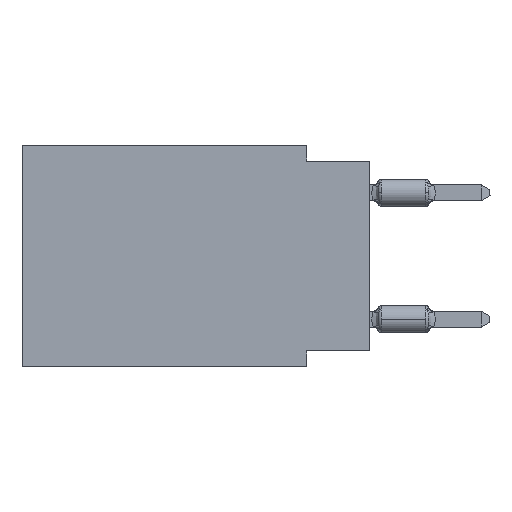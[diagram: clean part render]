
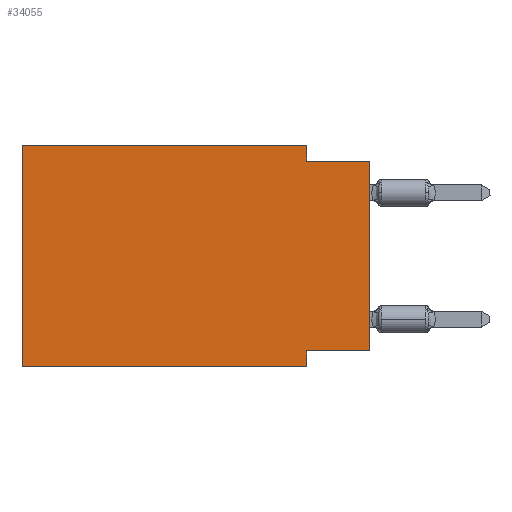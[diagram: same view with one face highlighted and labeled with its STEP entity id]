
A CAD part, left-side view. The second image highlights one B-rep face of the part: STEP entity #34055.
In plain terms, the highlighted planar face has unit normal (-1, 0, 0).
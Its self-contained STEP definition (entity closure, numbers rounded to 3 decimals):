
#623 = FACE_OUTER_BOUND ( 'NONE', #3907, .T. ) ;
#1321 = DIRECTION ( 'NONE',  ( 0., 0., -1. ) ) ;
#1369 = ORIENTED_EDGE ( 'NONE', *, *, #36295, .F. ) ;
#1447 = ORIENTED_EDGE ( 'NONE', *, *, #17365, .F. ) ;
#1953 = VERTEX_POINT ( 'NONE', #7689 ) ;
#2126 = DIRECTION ( 'NONE',  ( 0., 1., 0. ) ) ;
#2865 = VECTOR ( 'NONE', #28573, 1000. ) ;
#3158 = VERTEX_POINT ( 'NONE', #5037 ) ;
#3907 = EDGE_LOOP ( 'NONE', ( #31563, #3913, #12588, #1369, #12173, #6839, #1447, #6886 ) ) ;
#3913 = ORIENTED_EDGE ( 'NONE', *, *, #12245, .F. ) ;
#4157 = CARTESIAN_POINT ( 'NONE',  ( 0., 2.54, -0.635 ) ) ;
#4336 = LINE ( 'NONE', #18731, #15371 ) ;
#5037 = CARTESIAN_POINT ( 'NONE',  ( 0., 2.54, -8.255 ) ) ;
#5734 = LINE ( 'NONE', #35028, #26930 ) ;
#5789 = DIRECTION ( 'NONE',  ( 0., -1., 0. ) ) ;
#6024 = CARTESIAN_POINT ( 'NONE',  ( 0., 13.97, -8.89 ) ) ;
#6485 = CARTESIAN_POINT ( 'NONE',  ( 0., 0., 0. ) ) ;
#6839 = ORIENTED_EDGE ( 'NONE', *, *, #9500, .T. ) ;
#6886 = ORIENTED_EDGE ( 'NONE', *, *, #21259, .F. ) ;
#7689 = CARTESIAN_POINT ( 'NONE',  ( 0., 0., -0.635 ) ) ;
#7815 = EDGE_CURVE ( 'NONE', #43434, #20522, #46175, .T. ) ;
#9500 = EDGE_CURVE ( 'NONE', #43434, #27887, #12260, .T. ) ;
#9867 = DIRECTION ( 'NONE',  ( 0., 0., -1. ) ) ;
#10337 = LINE ( 'NONE', #28597, #28189 ) ;
#11064 = CARTESIAN_POINT ( 'NONE',  ( 0., 2.54, 0. ) ) ;
#12173 = ORIENTED_EDGE ( 'NONE', *, *, #7815, .F. ) ;
#12245 = EDGE_CURVE ( 'NONE', #22387, #1953, #4336, .T. ) ;
#12260 = LINE ( 'NONE', #6024, #30629 ) ;
#12588 = ORIENTED_EDGE ( 'NONE', *, *, #23973, .F. ) ;
#12964 = CARTESIAN_POINT ( 'NONE',  ( 0., 13.97, 0. ) ) ;
#15137 = LINE ( 'NONE', #11064, #46253 ) ;
#15371 = VECTOR ( 'NONE', #37236, 1000. ) ;
#17365 = EDGE_CURVE ( 'NONE', #3158, #27887, #10337, .T. ) ;
#18731 = CARTESIAN_POINT ( 'NONE',  ( 0., 0., -0.635 ) ) ;
#18931 = CARTESIAN_POINT ( 'NONE',  ( 0., 13.97, 0. ) ) ;
#20522 = VERTEX_POINT ( 'NONE', #18931 ) ;
#20640 = DIRECTION ( 'NONE',  ( 0., -1., 0. ) ) ;
#21259 = EDGE_CURVE ( 'NONE', #36828, #3158, #5734, .T. ) ;
#22072 = CARTESIAN_POINT ( 'NONE',  ( 0., 13.97, -8.89 ) ) ;
#22387 = VERTEX_POINT ( 'NONE', #4157 ) ;
#23973 = EDGE_CURVE ( 'NONE', #30638, #22387, #15137, .T. ) ;
#26930 = VECTOR ( 'NONE', #2126, 1000. ) ;
#27887 = VERTEX_POINT ( 'NONE', #29630 ) ;
#28189 = VECTOR ( 'NONE', #9867, 1000. ) ;
#28573 = DIRECTION ( 'NONE',  ( 0., 0., 1. ) ) ;
#28597 = CARTESIAN_POINT ( 'NONE',  ( 0., 2.54, -8.89 ) ) ;
#29630 = CARTESIAN_POINT ( 'NONE',  ( 0., 2.54, -8.89 ) ) ;
#30629 = VECTOR ( 'NONE', #5789, 1000. ) ;
#30638 = VERTEX_POINT ( 'NONE', #32525 ) ;
#31563 = ORIENTED_EDGE ( 'NONE', *, *, #43355, .T. ) ;
#32525 = CARTESIAN_POINT ( 'NONE',  ( 0., 2.54, 0. ) ) ;
#33769 = VECTOR ( 'NONE', #20640, 1000. ) ;
#34055 = ADVANCED_FACE ( 'NONE', ( #623 ), #45037, .F. ) ;
#34451 = CARTESIAN_POINT ( 'NONE',  ( 0., 13.97, 0. ) ) ;
#34904 = CARTESIAN_POINT ( 'NONE',  ( 0., 13.97, 0. ) ) ;
#35028 = CARTESIAN_POINT ( 'NONE',  ( 0., 0., -8.255 ) ) ;
#35079 = CARTESIAN_POINT ( 'NONE',  ( 0., 0., -8.255 ) ) ;
#36295 = EDGE_CURVE ( 'NONE', #20522, #30638, #42753, .T. ) ;
#36379 = AXIS2_PLACEMENT_3D ( 'NONE', #34451, #45264, #1321 ) ;
#36828 = VERTEX_POINT ( 'NONE', #35079 ) ;
#37236 = DIRECTION ( 'NONE',  ( 0., -1., 0. ) ) ;
#37476 = DIRECTION ( 'NONE',  ( 0., 0., -1. ) ) ;
#39630 = LINE ( 'NONE', #6485, #2865 ) ;
#42753 = LINE ( 'NONE', #12964, #33769 ) ;
#42817 = DIRECTION ( 'NONE',  ( 0., 0., 1. ) ) ;
#43355 = EDGE_CURVE ( 'NONE', #36828, #1953, #39630, .T. ) ;
#43434 = VERTEX_POINT ( 'NONE', #22072 ) ;
#45037 = PLANE ( 'NONE',  #36379 ) ;
#45264 = DIRECTION ( 'NONE',  ( 1., 0., 0. ) ) ;
#45821 = VECTOR ( 'NONE', #42817, 1000. ) ;
#46175 = LINE ( 'NONE', #34904, #45821 ) ;
#46253 = VECTOR ( 'NONE', #37476, 1000. ) ;
